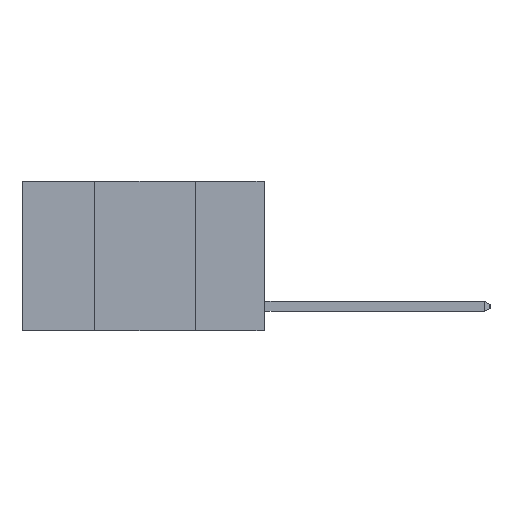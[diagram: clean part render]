
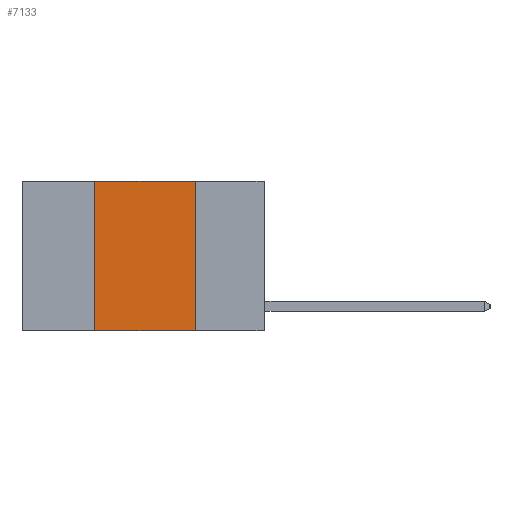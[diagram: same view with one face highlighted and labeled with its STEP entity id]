
A CAD part, left-side view. The second image highlights one B-rep face of the part: STEP entity #7133.
In plain terms, the highlighted planar face has unit normal (-1, 0, 0).
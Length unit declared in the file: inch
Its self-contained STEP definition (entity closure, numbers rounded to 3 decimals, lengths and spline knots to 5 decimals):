
#34 = DIRECTION ( 'NONE',  ( 1., 0., 0. ) ) ;
#86 = VECTOR ( 'NONE', #1526, 39.37008 ) ;
#617 = LINE ( 'NONE', #5284, #6549 ) ;
#874 = DIRECTION ( 'NONE',  ( 0., 0., -1. ) ) ;
#1088 = DIRECTION ( 'NONE',  ( 0., -1., 0. ) ) ;
#1322 = VERTEX_POINT ( 'NONE', #9691 ) ;
#1526 = DIRECTION ( 'NONE',  ( 0., 0., 1. ) ) ;
#2053 = VECTOR ( 'NONE', #1088, 39.37008 ) ;
#2921 = ORIENTED_EDGE ( 'NONE', *, *, #6058, .T. ) ;
#3278 = LINE ( 'NONE', #10580, #9662 ) ;
#3311 = CARTESIAN_POINT ( 'NONE',  ( 0., 0.17, -0.37 ) ) ;
#3827 = VERTEX_POINT ( 'NONE', #3311 ) ;
#3999 = DIRECTION ( 'NONE',  ( 0., -1., 0. ) ) ;
#4262 = CARTESIAN_POINT ( 'NONE',  ( 0., 0.17, 0. ) ) ;
#4349 = LINE ( 'NONE', #4625, #2053 ) ;
#4625 = CARTESIAN_POINT ( 'NONE',  ( 0., 0.6, 0. ) ) ;
#5284 = CARTESIAN_POINT ( 'NONE',  ( 0., 0.17, 0. ) ) ;
#5290 = EDGE_CURVE ( 'NONE', #1322, #8645, #4349, .T. ) ;
#5457 = PLANE ( 'NONE',  #8801 ) ;
#5691 = ORIENTED_EDGE ( 'NONE', *, *, #8588, .F. ) ;
#6058 = EDGE_CURVE ( 'NONE', #8453, #3827, #3278, .T. ) ;
#6318 = DIRECTION ( 'NONE',  ( 0., 0., -1. ) ) ;
#6549 = VECTOR ( 'NONE', #874, 39.37008 ) ;
#6975 = ORIENTED_EDGE ( 'NONE', *, *, #10872, .F. ) ;
#7133 = ADVANCED_FACE ( 'NONE', ( #7357 ), #5457, .F. ) ;
#7188 = LINE ( 'NONE', #9980, #86 ) ;
#7357 = FACE_OUTER_BOUND ( 'NONE', #9787, .T. ) ;
#7931 = CARTESIAN_POINT ( 'NONE',  ( 0., 0.6, 0. ) ) ;
#8193 = CARTESIAN_POINT ( 'NONE',  ( 0., 0.42, -0.37 ) ) ;
#8453 = VERTEX_POINT ( 'NONE', #8193 ) ;
#8588 = EDGE_CURVE ( 'NONE', #8453, #1322, #7188, .T. ) ;
#8645 = VERTEX_POINT ( 'NONE', #4262 ) ;
#8801 = AXIS2_PLACEMENT_3D ( 'NONE', #7931, #34, #6318 ) ;
#9662 = VECTOR ( 'NONE', #3999, 39.37008 ) ;
#9691 = CARTESIAN_POINT ( 'NONE',  ( 0., 0.42, 0. ) ) ;
#9787 = EDGE_LOOP ( 'NONE', ( #6975, #10155, #5691, #2921 ) ) ;
#9980 = CARTESIAN_POINT ( 'NONE',  ( 0., 0.42, 0. ) ) ;
#10155 = ORIENTED_EDGE ( 'NONE', *, *, #5290, .F. ) ;
#10580 = CARTESIAN_POINT ( 'NONE',  ( 0., 0.6, -0.37 ) ) ;
#10872 = EDGE_CURVE ( 'NONE', #8645, #3827, #617, .T. ) ;
